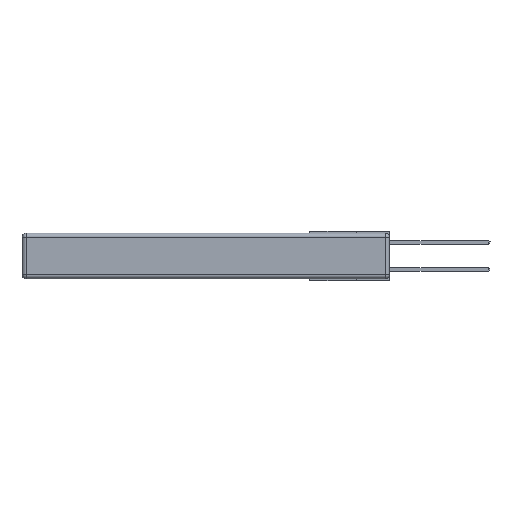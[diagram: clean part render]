
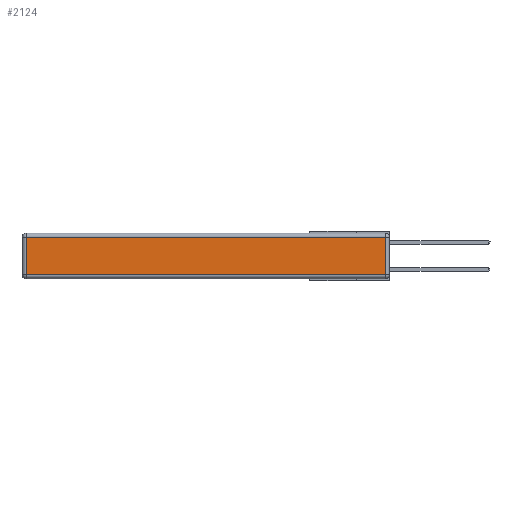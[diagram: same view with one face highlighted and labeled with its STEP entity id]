
A CAD part, left-side view. The second image highlights one B-rep face of the part: STEP entity #2124.
In plain terms, the highlighted planar face has unit normal (-1, 0, 0).
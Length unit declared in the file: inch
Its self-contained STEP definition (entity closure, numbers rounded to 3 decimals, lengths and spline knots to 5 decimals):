
#252 = FACE_OUTER_BOUND ( 'NONE', #2580, .T. ) ;
#317 = DIRECTION ( 'NONE',  ( -1., 0., 0. ) ) ;
#1162 = AXIS2_PLACEMENT_3D ( 'NONE', #7856, #317, #11600 ) ;
#1739 = ORIENTED_EDGE ( 'NONE', *, *, #4891, .T. ) ;
#1874 = VERTEX_POINT ( 'NONE', #12795 ) ;
#2124 = ADVANCED_FACE ( 'NONE', ( #252 ), #10296, .T. ) ;
#2375 = CARTESIAN_POINT ( 'NONE',  ( 0., 2.72, -0.343 ) ) ;
#2580 = EDGE_LOOP ( 'NONE', ( #10840, #11352, #8999, #1739 ) ) ;
#2639 = VERTEX_POINT ( 'NONE', #12206 ) ;
#2796 = CARTESIAN_POINT ( 'NONE',  ( 0., 0.03, -0.03 ) ) ;
#2984 = DIRECTION ( 'NONE',  ( 0., 0., 1. ) ) ;
#4108 = VERTEX_POINT ( 'NONE', #2796 ) ;
#4642 = DIRECTION ( 'NONE',  ( 0., -1., 0. ) ) ;
#4891 = EDGE_CURVE ( 'NONE', #2639, #6168, #12953, .T. ) ;
#5348 = CARTESIAN_POINT ( 'NONE',  ( 0., 2.72, -0.313 ) ) ;
#5662 = CARTESIAN_POINT ( 'NONE',  ( 0., 2.75, -0.03 ) ) ;
#6168 = VERTEX_POINT ( 'NONE', #5348 ) ;
#6555 = LINE ( 'NONE', #8606, #6907 ) ;
#6907 = VECTOR ( 'NONE', #2984, 39.37008 ) ;
#6993 = VECTOR ( 'NONE', #4642, 39.37008 ) ;
#7013 = CARTESIAN_POINT ( 'NONE',  ( 0., 0., -0.313 ) ) ;
#7856 = CARTESIAN_POINT ( 'NONE',  ( 0., 0., -0.343 ) ) ;
#8289 = EDGE_CURVE ( 'NONE', #4108, #2639, #11996, .T. ) ;
#8606 = CARTESIAN_POINT ( 'NONE',  ( 0., 0.03, -0.343 ) ) ;
#8999 = ORIENTED_EDGE ( 'NONE', *, *, #8289, .T. ) ;
#9321 = VECTOR ( 'NONE', #10112, 39.37008 ) ;
#9943 = VECTOR ( 'NONE', #10298, 39.37008 ) ;
#10112 = DIRECTION ( 'NONE',  ( 0., 1., 0. ) ) ;
#10296 = PLANE ( 'NONE',  #1162 ) ;
#10298 = DIRECTION ( 'NONE',  ( 0., 0., -1. ) ) ;
#10840 = ORIENTED_EDGE ( 'NONE', *, *, #12970, .T. ) ;
#10906 = EDGE_CURVE ( 'NONE', #1874, #4108, #6555, .T. ) ;
#11352 = ORIENTED_EDGE ( 'NONE', *, *, #10906, .T. ) ;
#11600 = DIRECTION ( 'NONE',  ( 0., 0., 1. ) ) ;
#11996 = LINE ( 'NONE', #5662, #9321 ) ;
#12206 = CARTESIAN_POINT ( 'NONE',  ( 0., 2.72, -0.03 ) ) ;
#12504 = LINE ( 'NONE', #7013, #6993 ) ;
#12795 = CARTESIAN_POINT ( 'NONE',  ( 0., 0.03, -0.313 ) ) ;
#12953 = LINE ( 'NONE', #2375, #9943 ) ;
#12970 = EDGE_CURVE ( 'NONE', #6168, #1874, #12504, .T. ) ;
